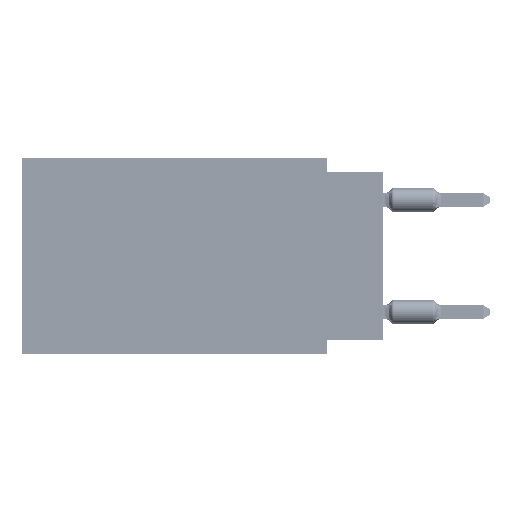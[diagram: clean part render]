
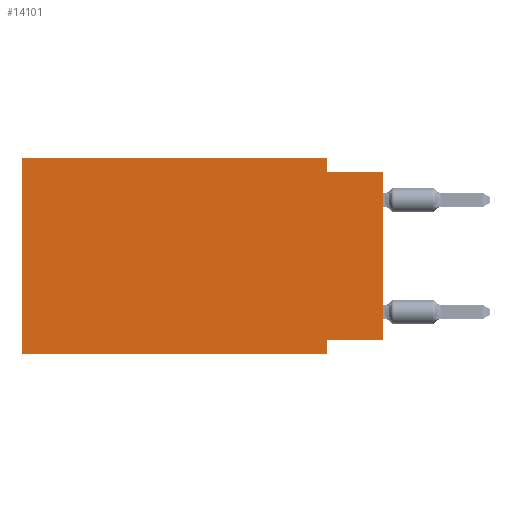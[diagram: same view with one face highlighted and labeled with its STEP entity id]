
A CAD part, left-side view. The second image highlights one B-rep face of the part: STEP entity #14101.
In plain terms, the highlighted planar face has unit normal (-1, 0, 0).
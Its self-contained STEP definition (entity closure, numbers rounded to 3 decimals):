
#2135 = VECTOR ( 'NONE', #49228, 1000. ) ;
#2499 = EDGE_CURVE ( 'NONE', #46287, #16906, #51279, .T. ) ;
#3500 = DIRECTION ( 'NONE',  ( 1., 0., 0. ) ) ;
#3763 = CARTESIAN_POINT ( 'NONE',  ( 0., 0., -0.635 ) ) ;
#6085 = CARTESIAN_POINT ( 'NONE',  ( 0., 16.383, -8.89 ) ) ;
#9209 = DIRECTION ( 'NONE',  ( 0., 1., 0. ) ) ;
#9515 = ORIENTED_EDGE ( 'NONE', *, *, #15974, .T. ) ;
#10866 = VECTOR ( 'NONE', #13275, 1000. ) ;
#11206 = LINE ( 'NONE', #6085, #56291 ) ;
#12210 = ORIENTED_EDGE ( 'NONE', *, *, #2499, .F. ) ;
#12832 = VERTEX_POINT ( 'NONE', #23698 ) ;
#13275 = DIRECTION ( 'NONE',  ( 0., 0., -1. ) ) ;
#14101 = ADVANCED_FACE ( 'NONE', ( #60639 ), #55519, .F. ) ;
#14265 = LINE ( 'NONE', #19405, #2135 ) ;
#15974 = EDGE_CURVE ( 'NONE', #50020, #64880, #52494, .T. ) ;
#16515 = EDGE_CURVE ( 'NONE', #63264, #12832, #28693, .T. ) ;
#16906 = VERTEX_POINT ( 'NONE', #19331 ) ;
#19331 = CARTESIAN_POINT ( 'NONE',  ( 0., 2.54, -8.89 ) ) ;
#19405 = CARTESIAN_POINT ( 'NONE',  ( 0., 16.383, 0. ) ) ;
#20301 = ORIENTED_EDGE ( 'NONE', *, *, #16515, .F. ) ;
#22739 = ORIENTED_EDGE ( 'NONE', *, *, #42342, .F. ) ;
#23698 = CARTESIAN_POINT ( 'NONE',  ( 0., 2.54, -0.635 ) ) ;
#24032 = CARTESIAN_POINT ( 'NONE',  ( 0., 0., -8.255 ) ) ;
#27732 = CARTESIAN_POINT ( 'NONE',  ( 0., 0., -0.635 ) ) ;
#28693 = LINE ( 'NONE', #56008, #10866 ) ;
#29111 = CARTESIAN_POINT ( 'NONE',  ( 0., 2.54, -8.255 ) ) ;
#29518 = CARTESIAN_POINT ( 'NONE',  ( 0., 16.383, 0. ) ) ;
#31514 = ORIENTED_EDGE ( 'NONE', *, *, #52733, .T. ) ;
#31879 = ORIENTED_EDGE ( 'NONE', *, *, #59087, .F. ) ;
#32840 = LINE ( 'NONE', #42771, #59001 ) ;
#34470 = LINE ( 'NONE', #27732, #61911 ) ;
#36415 = EDGE_CURVE ( 'NONE', #56197, #63264, #32840, .T. ) ;
#37095 = DIRECTION ( 'NONE',  ( 0., 0., 1. ) ) ;
#37556 = VECTOR ( 'NONE', #65989, 1000. ) ;
#38249 = DIRECTION ( 'NONE',  ( 0., -1., 0. ) ) ;
#38641 = EDGE_LOOP ( 'NONE', ( #9515, #62605, #20301, #45052, #31879, #31514, #12210, #22739 ) ) ;
#40624 = CARTESIAN_POINT ( 'NONE',  ( 0., 16.383, -8.89 ) ) ;
#41140 = CARTESIAN_POINT ( 'NONE',  ( 0., 2.54, 0. ) ) ;
#41368 = VECTOR ( 'NONE', #37095, 1000. ) ;
#42342 = EDGE_CURVE ( 'NONE', #50020, #46287, #51295, .T. ) ;
#42771 = CARTESIAN_POINT ( 'NONE',  ( 0., 16.383, 0. ) ) ;
#43128 = DIRECTION ( 'NONE',  ( 0., -1., 0. ) ) ;
#43251 = CARTESIAN_POINT ( 'NONE',  ( 0., 0., 0. ) ) ;
#44460 = VECTOR ( 'NONE', #9209, 1000. ) ;
#45052 = ORIENTED_EDGE ( 'NONE', *, *, #36415, .F. ) ;
#46287 = VERTEX_POINT ( 'NONE', #29111 ) ;
#49228 = DIRECTION ( 'NONE',  ( 0., 0., 1. ) ) ;
#49964 = CARTESIAN_POINT ( 'NONE',  ( 0., 2.54, -8.89 ) ) ;
#50020 = VERTEX_POINT ( 'NONE', #24032 ) ;
#50714 = DIRECTION ( 'NONE',  ( 0., 0., -1. ) ) ;
#51279 = LINE ( 'NONE', #49964, #37556 ) ;
#51295 = LINE ( 'NONE', #67002, #44460 ) ;
#52494 = LINE ( 'NONE', #43251, #41368 ) ;
#52733 = EDGE_CURVE ( 'NONE', #59275, #16906, #11206, .T. ) ;
#53709 = DIRECTION ( 'NONE',  ( 0., -1., 0. ) ) ;
#54102 = EDGE_CURVE ( 'NONE', #12832, #64880, #34470, .T. ) ;
#54592 = CARTESIAN_POINT ( 'NONE',  ( 0., 16.383, 0. ) ) ;
#55519 = PLANE ( 'NONE',  #61229 ) ;
#56008 = CARTESIAN_POINT ( 'NONE',  ( 0., 2.54, 0. ) ) ;
#56197 = VERTEX_POINT ( 'NONE', #54592 ) ;
#56291 = VECTOR ( 'NONE', #38249, 1000. ) ;
#59001 = VECTOR ( 'NONE', #53709, 1000. ) ;
#59087 = EDGE_CURVE ( 'NONE', #59275, #56197, #14265, .T. ) ;
#59275 = VERTEX_POINT ( 'NONE', #40624 ) ;
#60639 = FACE_OUTER_BOUND ( 'NONE', #38641, .T. ) ;
#61229 = AXIS2_PLACEMENT_3D ( 'NONE', #29518, #3500, #50714 ) ;
#61911 = VECTOR ( 'NONE', #43128, 1000. ) ;
#62605 = ORIENTED_EDGE ( 'NONE', *, *, #54102, .F. ) ;
#63264 = VERTEX_POINT ( 'NONE', #41140 ) ;
#64880 = VERTEX_POINT ( 'NONE', #3763 ) ;
#65989 = DIRECTION ( 'NONE',  ( 0., 0., -1. ) ) ;
#67002 = CARTESIAN_POINT ( 'NONE',  ( 0., 0., -8.255 ) ) ;
